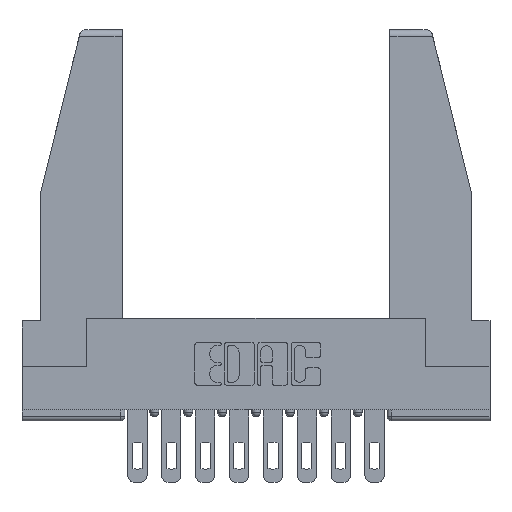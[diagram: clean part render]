
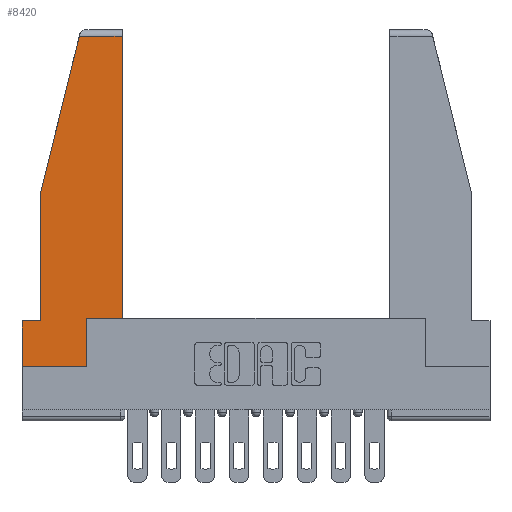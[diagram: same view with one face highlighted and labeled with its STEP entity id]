
A CAD part, top view. The second image highlights one B-rep face of the part: STEP entity #8420.
In plain terms, the highlighted planar face has unit normal (0, 0, 1).
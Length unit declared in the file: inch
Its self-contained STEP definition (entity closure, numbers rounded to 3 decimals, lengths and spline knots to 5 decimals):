
#93 = VECTOR ( 'NONE', #11873, 39.37008 ) ;
#99 = VECTOR ( 'NONE', #4195, 39.37008 ) ;
#202 = CARTESIAN_POINT ( 'NONE',  ( 0.461, 0.223, 0. ) ) ;
#299 = EDGE_CURVE ( 'NONE', #8416, #7303, #1793, .T. ) ;
#571 = LINE ( 'NONE', #1731, #4351 ) ;
#987 = VERTEX_POINT ( 'NONE', #9426 ) ;
#1036 = ORIENTED_EDGE ( 'NONE', *, *, #12483, .T. ) ;
#1146 = DIRECTION ( 'NONE',  ( 1., 0., 0. ) ) ;
#1364 = VERTEX_POINT ( 'NONE', #6659 ) ;
#1571 = LINE ( 'NONE', #8657, #93 ) ;
#1728 = CARTESIAN_POINT ( 'NONE',  ( 0., 1.52, 0. ) ) ;
#1731 = CARTESIAN_POINT ( 'NONE',  ( 0.297, 0., 0. ) ) ;
#1793 = LINE ( 'NONE', #1728, #10124 ) ;
#1876 = VERTEX_POINT ( 'NONE', #202 ) ;
#2079 = AXIS2_PLACEMENT_3D ( 'NONE', #4450, #5275, #1146 ) ;
#2092 = CARTESIAN_POINT ( 'NONE',  ( 0.086, 0.8, 0. ) ) ;
#2452 = CARTESIAN_POINT ( 'NONE',  ( 0., 0.21, 0. ) ) ;
#2719 = VERTEX_POINT ( 'NONE', #4028 ) ;
#2847 = VERTEX_POINT ( 'NONE', #8023 ) ;
#3048 = VECTOR ( 'NONE', #3216, 39.37008 ) ;
#3216 = DIRECTION ( 'NONE',  ( 0., -1., 0. ) ) ;
#3236 = CARTESIAN_POINT ( 'NONE',  ( 0.461, 0.223, 0. ) ) ;
#3565 = FACE_OUTER_BOUND ( 'NONE', #7438, .T. ) ;
#3650 = DIRECTION ( 'NONE',  ( 1., 0., 0. ) ) ;
#4028 = CARTESIAN_POINT ( 'NONE',  ( 0.086, 0.8, 0. ) ) ;
#4033 = LINE ( 'NONE', #2452, #9580 ) ;
#4195 = DIRECTION ( 'NONE',  ( 0., 1., 0. ) ) ;
#4196 = EDGE_CURVE ( 'NONE', #987, #1876, #8733, .T. ) ;
#4351 = VECTOR ( 'NONE', #7868, 39.37008 ) ;
#4450 = CARTESIAN_POINT ( 'NONE',  ( 0., 0., 0. ) ) ;
#4703 = CARTESIAN_POINT ( 'NONE',  ( 0.297, 0.223, 0. ) ) ;
#5275 = DIRECTION ( 'NONE',  ( 0., 0., 1. ) ) ;
#5567 = ORIENTED_EDGE ( 'NONE', *, *, #12051, .T. ) ;
#5814 = CARTESIAN_POINT ( 'NONE',  ( 0., 0., 0. ) ) ;
#5955 = EDGE_CURVE ( 'NONE', #2719, #6993, #13369, .T. ) ;
#6152 = LINE ( 'NONE', #9674, #9406 ) ;
#6172 = DIRECTION ( 'NONE',  ( 0., -1., 0. ) ) ;
#6600 = CARTESIAN_POINT ( 'NONE',  ( 0.2636, 1.52, 0. ) ) ;
#6658 = ORIENTED_EDGE ( 'NONE', *, *, #8965, .T. ) ;
#6659 = CARTESIAN_POINT ( 'NONE',  ( 0.297, 0., 0. ) ) ;
#6825 = ORIENTED_EDGE ( 'NONE', *, *, #299, .T. ) ;
#6993 = VERTEX_POINT ( 'NONE', #10278 ) ;
#7303 = VERTEX_POINT ( 'NONE', #6600 ) ;
#7438 = EDGE_LOOP ( 'NONE', ( #6658, #6825, #11592, #10863, #7471, #1036, #5567, #9925, #8448 ) ) ;
#7471 = ORIENTED_EDGE ( 'NONE', *, *, #11942, .T. ) ;
#7868 = DIRECTION ( 'NONE',  ( 0., 1., 0. ) ) ;
#8023 = CARTESIAN_POINT ( 'NONE',  ( 0., 0.21, 0. ) ) ;
#8249 = VECTOR ( 'NONE', #3650, 39.37008 ) ;
#8263 = LINE ( 'NONE', #11670, #3048 ) ;
#8416 = VERTEX_POINT ( 'NONE', #10498 ) ;
#8420 = ADVANCED_FACE ( 'NONE', ( #3565 ), #10673, .T. ) ;
#8448 = ORIENTED_EDGE ( 'NONE', *, *, #4196, .T. ) ;
#8657 = CARTESIAN_POINT ( 'NONE',  ( 0., 0., 0. ) ) ;
#8733 = LINE ( 'NONE', #4703, #8249 ) ;
#8965 = EDGE_CURVE ( 'NONE', #1876, #8416, #13284, .T. ) ;
#9149 = EDGE_CURVE ( 'NONE', #7303, #2719, #6152, .T. ) ;
#9190 = VECTOR ( 'NONE', #6172, 39.37008 ) ;
#9406 = VECTOR ( 'NONE', #10623, 39.37008 ) ;
#9426 = CARTESIAN_POINT ( 'NONE',  ( 0.297, 0.223, 0. ) ) ;
#9580 = VECTOR ( 'NONE', #9704, 39.37008 ) ;
#9674 = CARTESIAN_POINT ( 'NONE',  ( 0.271, 1.55, 0. ) ) ;
#9704 = DIRECTION ( 'NONE',  ( -1., 0., 0. ) ) ;
#9925 = ORIENTED_EDGE ( 'NONE', *, *, #11582, .T. ) ;
#10124 = VECTOR ( 'NONE', #13002, 39.37008 ) ;
#10278 = CARTESIAN_POINT ( 'NONE',  ( 0.086, 0.21, 0. ) ) ;
#10498 = CARTESIAN_POINT ( 'NONE',  ( 0.461, 1.52, 0. ) ) ;
#10623 = DIRECTION ( 'NONE',  ( -0.239, -0.971, 0. ) ) ;
#10673 = PLANE ( 'NONE',  #2079 ) ;
#10863 = ORIENTED_EDGE ( 'NONE', *, *, #5955, .T. ) ;
#11046 = VERTEX_POINT ( 'NONE', #5814 ) ;
#11582 = EDGE_CURVE ( 'NONE', #1364, #987, #571, .T. ) ;
#11592 = ORIENTED_EDGE ( 'NONE', *, *, #9149, .T. ) ;
#11670 = CARTESIAN_POINT ( 'NONE',  ( 0., 0.21, 0. ) ) ;
#11873 = DIRECTION ( 'NONE',  ( 1., 0., 0. ) ) ;
#11942 = EDGE_CURVE ( 'NONE', #6993, #2847, #4033, .T. ) ;
#12051 = EDGE_CURVE ( 'NONE', #11046, #1364, #1571, .T. ) ;
#12483 = EDGE_CURVE ( 'NONE', #2847, #11046, #8263, .T. ) ;
#13002 = DIRECTION ( 'NONE',  ( -1., 0., 0. ) ) ;
#13284 = LINE ( 'NONE', #3236, #99 ) ;
#13369 = LINE ( 'NONE', #2092, #9190 ) ;
